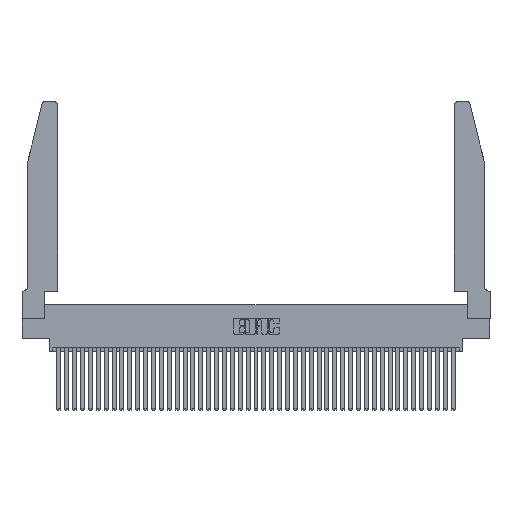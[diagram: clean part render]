
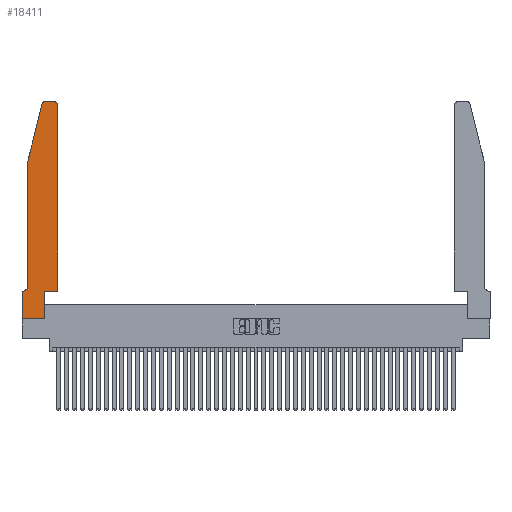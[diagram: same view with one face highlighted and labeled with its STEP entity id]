
A CAD part, top view. The second image highlights one B-rep face of the part: STEP entity #18411.
In plain terms, the highlighted planar face has unit normal (0, 0, 1).
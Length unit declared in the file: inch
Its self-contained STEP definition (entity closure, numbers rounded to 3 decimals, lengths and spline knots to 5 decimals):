
#204 = VECTOR ( 'NONE', #39814, 39.37008 ) ;
#318 = ORIENTED_EDGE ( 'NONE', *, *, #28320, .T. ) ;
#1425 = VERTEX_POINT ( 'NONE', #35118 ) ;
#2003 = ORIENTED_EDGE ( 'NONE', *, *, #42982, .T. ) ;
#3983 = EDGE_CURVE ( 'NONE', #14450, #22661, #11810, .T. ) ;
#4385 = DIRECTION ( 'NONE',  ( -1., 0., 0. ) ) ;
#4652 = EDGE_CURVE ( 'NONE', #42232, #29618, #10201, .T. ) ;
#4880 = ORIENTED_EDGE ( 'NONE', *, *, #14672, .T. ) ;
#5676 = VECTOR ( 'NONE', #41269, 39.37008 ) ;
#5705 = LINE ( 'NONE', #30894, #12568 ) ;
#5835 = DIRECTION ( 'NONE',  ( 1., 0., 0. ) ) ;
#6259 = EDGE_CURVE ( 'NONE', #17536, #11928, #6332, .T. ) ;
#6332 = LINE ( 'NONE', #9007, #19477 ) ;
#7278 = EDGE_CURVE ( 'NONE', #29562, #23368, #38236, .T. ) ;
#7610 = CARTESIAN_POINT ( 'NONE',  ( 0.0755, 2., 0.37 ) ) ;
#7677 = DIRECTION ( 'NONE',  ( 1., 0., 0. ) ) ;
#7925 = CARTESIAN_POINT ( 'NONE',  ( 0.0755, 0.35, 0.37 ) ) ;
#7958 = VERTEX_POINT ( 'NONE', #18251 ) ;
#8272 = CARTESIAN_POINT ( 'NONE',  ( 0.284, 2.75, 0.37 ) ) ;
#9007 = CARTESIAN_POINT ( 'NONE',  ( 0.4505, 0.35, 0.37 ) ) ;
#9268 = LINE ( 'NONE', #7925, #35584 ) ;
#9356 = PLANE ( 'NONE',  #38390 ) ;
#9495 = CARTESIAN_POINT ( 'NONE',  ( 0., 0.35, 0.37 ) ) ;
#10002 = CARTESIAN_POINT ( 'NONE',  ( 0.4205, 2.75, 0.37 ) ) ;
#10201 = LINE ( 'NONE', #18346, #24341 ) ;
#10460 = EDGE_CURVE ( 'NONE', #7958, #27980, #19509, .T. ) ;
#11810 = LINE ( 'NONE', #12505, #204 ) ;
#11905 = CARTESIAN_POINT ( 'NONE',  ( 0.0055, 0.42, 0.37 ) ) ;
#11928 = VERTEX_POINT ( 'NONE', #13554 ) ;
#12505 = CARTESIAN_POINT ( 'NONE',  ( 0.2865, 0.35, 0.37 ) ) ;
#12568 = VECTOR ( 'NONE', #7677, 39.37008 ) ;
#12571 = AXIS2_PLACEMENT_3D ( 'NONE', #17424, #31708, #5835 ) ;
#12712 = EDGE_CURVE ( 'NONE', #23161, #1425, #38323, .T. ) ;
#13253 = ORIENTED_EDGE ( 'NONE', *, *, #3983, .T. ) ;
#13349 = VECTOR ( 'NONE', #18887, 39.37008 ) ;
#13554 = CARTESIAN_POINT ( 'NONE',  ( 0.4505, 2.72, 0.37 ) ) ;
#13587 = AXIS2_PLACEMENT_3D ( 'NONE', #17829, #17976, #38309 ) ;
#14450 = VERTEX_POINT ( 'NONE', #27943 ) ;
#14672 = EDGE_CURVE ( 'NONE', #23368, #14450, #5705, .T. ) ;
#14849 = CARTESIAN_POINT ( 'NONE',  ( 0.4505, 0.35, 0.37 ) ) ;
#14991 = VECTOR ( 'NONE', #17197, 39.37008 ) ;
#14998 = DIRECTION ( 'NONE',  ( -1., 0., 0. ) ) ;
#15217 = ORIENTED_EDGE ( 'NONE', *, *, #7278, .T. ) ;
#15273 = DIRECTION ( 'NONE',  ( 0., 0., -1. ) ) ;
#16741 = CIRCLE ( 'NONE', #13587, 0.03 ) ;
#17029 = ORIENTED_EDGE ( 'NONE', *, *, #26868, .T. ) ;
#17197 = DIRECTION ( 'NONE',  ( 0., -1., 0. ) ) ;
#17424 = CARTESIAN_POINT ( 'NONE',  ( 0.284, 2.72, 0.37 ) ) ;
#17536 = VERTEX_POINT ( 'NONE', #14849 ) ;
#17829 = CARTESIAN_POINT ( 'NONE',  ( 0.4205, 2.72, 0.37 ) ) ;
#17976 = DIRECTION ( 'NONE',  ( 0., 0., 1. ) ) ;
#18251 = CARTESIAN_POINT ( 'NONE',  ( 0.0755, 0.42, 0.37 ) ) ;
#18298 = EDGE_CURVE ( 'NONE', #22661, #17536, #35476, .T. ) ;
#18346 = CARTESIAN_POINT ( 'NONE',  ( 0.2605, 2.75, 0.37 ) ) ;
#18411 = ADVANCED_FACE ( 'NONE', ( #27577 ), #9356, .T. ) ;
#18887 = DIRECTION ( 'NONE',  ( 1., 0., 0. ) ) ;
#19477 = VECTOR ( 'NONE', #39275, 39.37008 ) ;
#19509 = CIRCLE ( 'NONE', #31148, 0.07 ) ;
#20281 = CARTESIAN_POINT ( 'NONE',  ( 0.0755, 2., 0.37 ) ) ;
#21234 = CARTESIAN_POINT ( 'NONE',  ( 0.25487, 2.72718, 0.37 ) ) ;
#22661 = VERTEX_POINT ( 'NONE', #41834 ) ;
#23139 = ORIENTED_EDGE ( 'NONE', *, *, #18298, .T. ) ;
#23161 = VERTEX_POINT ( 'NONE', #21234 ) ;
#23368 = VERTEX_POINT ( 'NONE', #27676 ) ;
#24341 = VECTOR ( 'NONE', #32183, 39.37008 ) ;
#25465 = CIRCLE ( 'NONE', #12571, 0.03 ) ;
#25494 = LINE ( 'NONE', #20281, #14991 ) ;
#25751 = ORIENTED_EDGE ( 'NONE', *, *, #33277, .T. ) ;
#26868 = EDGE_CURVE ( 'NONE', #11928, #42232, #16741, .T. ) ;
#27514 = ORIENTED_EDGE ( 'NONE', *, *, #10460, .T. ) ;
#27577 = FACE_OUTER_BOUND ( 'NONE', #32984, .T. ) ;
#27676 = CARTESIAN_POINT ( 'NONE',  ( 0., 0., 0.37 ) ) ;
#27943 = CARTESIAN_POINT ( 'NONE',  ( 0.2865, 0., 0.37 ) ) ;
#27980 = VERTEX_POINT ( 'NONE', #43360 ) ;
#28320 = EDGE_CURVE ( 'NONE', #27980, #29562, #9268, .T. ) ;
#29156 = ORIENTED_EDGE ( 'NONE', *, *, #12712, .T. ) ;
#29562 = VERTEX_POINT ( 'NONE', #42213 ) ;
#29618 = VERTEX_POINT ( 'NONE', #8272 ) ;
#30894 = CARTESIAN_POINT ( 'NONE',  ( 0., 0., 0.37 ) ) ;
#31148 = AXIS2_PLACEMENT_3D ( 'NONE', #11905, #15273, #14998 ) ;
#31708 = DIRECTION ( 'NONE',  ( 0., 0., 1. ) ) ;
#32183 = DIRECTION ( 'NONE',  ( -1., 0., 0. ) ) ;
#32294 = DIRECTION ( 'NONE',  ( 0., -1., 0. ) ) ;
#32984 = EDGE_LOOP ( 'NONE', ( #39211, #2003, #29156, #25751, #27514, #318, #15217, #4880, #13253, #23139, #34816, #17029 ) ) ;
#33277 = EDGE_CURVE ( 'NONE', #1425, #7958, #25494, .T. ) ;
#34816 = ORIENTED_EDGE ( 'NONE', *, *, #6259, .T. ) ;
#35118 = CARTESIAN_POINT ( 'NONE',  ( 0.0755, 2., 0.37 ) ) ;
#35476 = LINE ( 'NONE', #42135, #13349 ) ;
#35584 = VECTOR ( 'NONE', #4385, 39.37008 ) ;
#35607 = VECTOR ( 'NONE', #32294, 39.37008 ) ;
#35675 = DIRECTION ( 'NONE',  ( 0., 0., 1. ) ) ;
#38236 = LINE ( 'NONE', #39047, #35607 ) ;
#38309 = DIRECTION ( 'NONE',  ( 1., 0., 0. ) ) ;
#38323 = LINE ( 'NONE', #7610, #5676 ) ;
#38390 = AXIS2_PLACEMENT_3D ( 'NONE', #9495, #35675, #42426 ) ;
#39047 = CARTESIAN_POINT ( 'NONE',  ( 0., 0., 0.37 ) ) ;
#39211 = ORIENTED_EDGE ( 'NONE', *, *, #4652, .T. ) ;
#39275 = DIRECTION ( 'NONE',  ( 0., 1., 0. ) ) ;
#39814 = DIRECTION ( 'NONE',  ( 0., 1., 0. ) ) ;
#41269 = DIRECTION ( 'NONE',  ( -0.239, -0.971, 0. ) ) ;
#41834 = CARTESIAN_POINT ( 'NONE',  ( 0.2865, 0.35, 0.37 ) ) ;
#42135 = CARTESIAN_POINT ( 'NONE',  ( 0.4505, 0.35, 0.37 ) ) ;
#42213 = CARTESIAN_POINT ( 'NONE',  ( 0., 0.35, 0.37 ) ) ;
#42232 = VERTEX_POINT ( 'NONE', #10002 ) ;
#42426 = DIRECTION ( 'NONE',  ( 1., 0., 0. ) ) ;
#42982 = EDGE_CURVE ( 'NONE', #29618, #23161, #25465, .T. ) ;
#43360 = CARTESIAN_POINT ( 'NONE',  ( 0.0055, 0.35, 0.37 ) ) ;
